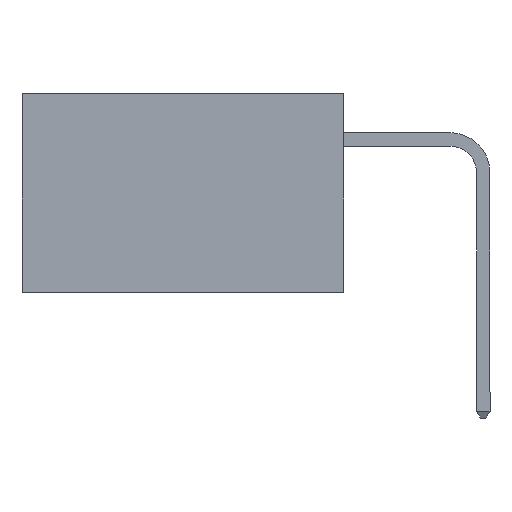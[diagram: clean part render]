
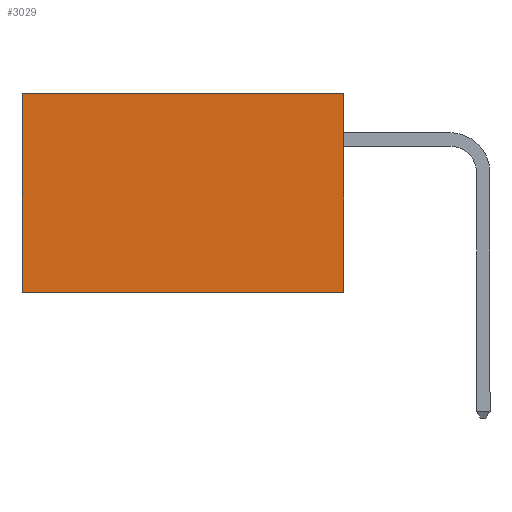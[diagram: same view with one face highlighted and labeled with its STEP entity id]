
A CAD part, left-side view. The second image highlights one B-rep face of the part: STEP entity #3029.
In plain terms, the highlighted planar face has unit normal (-1, 0, 0).
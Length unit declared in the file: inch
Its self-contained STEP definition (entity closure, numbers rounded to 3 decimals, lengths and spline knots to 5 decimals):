
#82 = DIRECTION ( 'NONE',  ( 0., 1., 0. ) ) ;
#220 = CARTESIAN_POINT ( 'NONE',  ( 0.298, 0., -0.37 ) ) ;
#351 = ORIENTED_EDGE ( 'NONE', *, *, #2121, .F. ) ;
#620 = VECTOR ( 'NONE', #82, 39.37008 ) ;
#1427 = EDGE_CURVE ( 'NONE', #2684, #5264, #3375, .T. ) ;
#1872 = DIRECTION ( 'NONE',  ( 0., 1., 0. ) ) ;
#2002 = ORIENTED_EDGE ( 'NONE', *, *, #1427, .T. ) ;
#2038 = DIRECTION ( 'NONE',  ( 0., 0., -1. ) ) ;
#2121 = EDGE_CURVE ( 'NONE', #5167, #4390, #3014, .T. ) ;
#2272 = CARTESIAN_POINT ( 'NONE',  ( 0.298, 0., 0. ) ) ;
#2684 = VERTEX_POINT ( 'NONE', #8400 ) ;
#2759 = ORIENTED_EDGE ( 'NONE', *, *, #6541, .F. ) ;
#3014 = LINE ( 'NONE', #220, #620 ) ;
#3029 = ADVANCED_FACE ( 'NONE', ( #7117 ), #7174, .F. ) ;
#3375 = LINE ( 'NONE', #6879, #9582 ) ;
#3889 = CARTESIAN_POINT ( 'NONE',  ( 0.298, 0., 0. ) ) ;
#4016 = CARTESIAN_POINT ( 'NONE',  ( 0.298, 0.6, 0. ) ) ;
#4156 = LINE ( 'NONE', #6211, #8469 ) ;
#4252 = LINE ( 'NONE', #3889, #8311 ) ;
#4390 = VERTEX_POINT ( 'NONE', #7472 ) ;
#4601 = DIRECTION ( 'NONE',  ( 0., 0., -1. ) ) ;
#4884 = AXIS2_PLACEMENT_3D ( 'NONE', #2272, #7762, #4601 ) ;
#5080 = EDGE_CURVE ( 'NONE', #5264, #4390, #4156, .T. ) ;
#5167 = VERTEX_POINT ( 'NONE', #6371 ) ;
#5264 = VERTEX_POINT ( 'NONE', #4016 ) ;
#6211 = CARTESIAN_POINT ( 'NONE',  ( 0.298, 0.6, 0. ) ) ;
#6371 = CARTESIAN_POINT ( 'NONE',  ( 0.298, 0., -0.37 ) ) ;
#6541 = EDGE_CURVE ( 'NONE', #2684, #5167, #4252, .T. ) ;
#6879 = CARTESIAN_POINT ( 'NONE',  ( 0.298, 0., 0. ) ) ;
#7117 = FACE_OUTER_BOUND ( 'NONE', #10730, .T. ) ;
#7174 = PLANE ( 'NONE',  #4884 ) ;
#7472 = CARTESIAN_POINT ( 'NONE',  ( 0.298, 0.6, -0.37 ) ) ;
#7762 = DIRECTION ( 'NONE',  ( 1., 0., 0. ) ) ;
#7788 = ORIENTED_EDGE ( 'NONE', *, *, #5080, .T. ) ;
#8311 = VECTOR ( 'NONE', #2038, 39.37008 ) ;
#8400 = CARTESIAN_POINT ( 'NONE',  ( 0.298, 0., 0. ) ) ;
#8469 = VECTOR ( 'NONE', #9697, 39.37008 ) ;
#9582 = VECTOR ( 'NONE', #1872, 39.37008 ) ;
#9697 = DIRECTION ( 'NONE',  ( 0., 0., -1. ) ) ;
#10730 = EDGE_LOOP ( 'NONE', ( #7788, #351, #2759, #2002 ) ) ;
